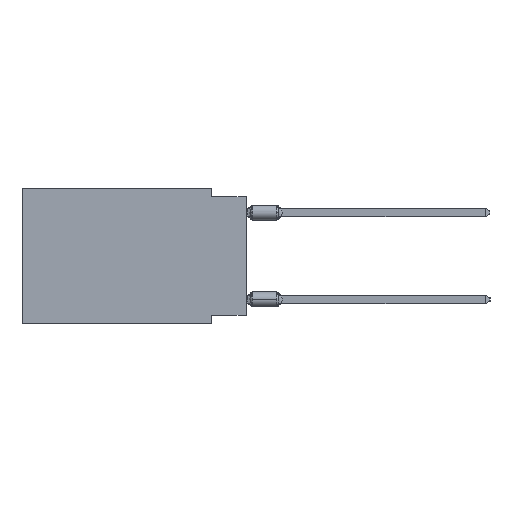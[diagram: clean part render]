
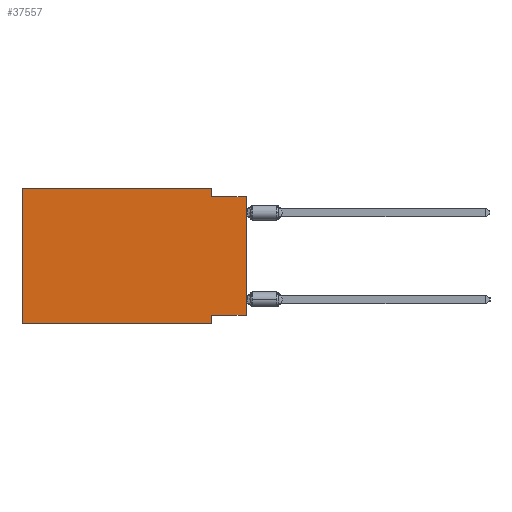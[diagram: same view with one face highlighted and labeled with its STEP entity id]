
A CAD part, left-side view. The second image highlights one B-rep face of the part: STEP entity #37557.
In plain terms, the highlighted planar face has unit normal (-1, 0, 0).
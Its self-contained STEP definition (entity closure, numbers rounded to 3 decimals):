
#1006 = VECTOR ( 'NONE', #11086, 1000. ) ;
#1692 = VECTOR ( 'NONE', #4965, 1000. ) ;
#1946 = PLANE ( 'NONE',  #30119 ) ;
#2645 = LINE ( 'NONE', #5754, #31853 ) ;
#2803 = CARTESIAN_POINT ( 'NONE',  ( 0., 16.383, 0. ) ) ;
#3024 = EDGE_CURVE ( 'NONE', #30024, #15613, #28320, .T. ) ;
#3860 = CARTESIAN_POINT ( 'NONE',  ( 0., 2.54, -9.271 ) ) ;
#4037 = DIRECTION ( 'NONE',  ( 0., 1., 0. ) ) ;
#4965 = DIRECTION ( 'NONE',  ( 0., 0., 1. ) ) ;
#5754 = CARTESIAN_POINT ( 'NONE',  ( 0., 0., -0.635 ) ) ;
#6241 = ORIENTED_EDGE ( 'NONE', *, *, #9407, .F. ) ;
#6508 = VECTOR ( 'NONE', #21291, 1000. ) ;
#6972 = ORIENTED_EDGE ( 'NONE', *, *, #30309, .F. ) ;
#7130 = ORIENTED_EDGE ( 'NONE', *, *, #29194, .T. ) ;
#7283 = VERTEX_POINT ( 'NONE', #7857 ) ;
#7857 = CARTESIAN_POINT ( 'NONE',  ( 0., 16.383, 0. ) ) ;
#8358 = VERTEX_POINT ( 'NONE', #12659 ) ;
#8396 = VECTOR ( 'NONE', #17007, 1000. ) ;
#8536 = DIRECTION ( 'NONE',  ( 1., 0., 0. ) ) ;
#8633 = EDGE_LOOP ( 'NONE', ( #27530, #24443, #30671, #10211, #6972, #7130, #30301, #6241 ) ) ;
#9407 = EDGE_CURVE ( 'NONE', #30024, #36001, #18699, .T. ) ;
#10211 = ORIENTED_EDGE ( 'NONE', *, *, #33633, .F. ) ;
#11086 = DIRECTION ( 'NONE',  ( 0., 0., 1. ) ) ;
#11648 = CARTESIAN_POINT ( 'NONE',  ( 0., 2.54, -0.635 ) ) ;
#12659 = CARTESIAN_POINT ( 'NONE',  ( 0., 16.383, -9.906 ) ) ;
#14315 = FACE_OUTER_BOUND ( 'NONE', #8633, .T. ) ;
#14510 = CARTESIAN_POINT ( 'NONE',  ( 0., 16.383, 0. ) ) ;
#14517 = VECTOR ( 'NONE', #34307, 1000. ) ;
#14641 = DIRECTION ( 'NONE',  ( 0., -1., 0. ) ) ;
#15522 = VERTEX_POINT ( 'NONE', #22913 ) ;
#15613 = VERTEX_POINT ( 'NONE', #26211 ) ;
#17007 = DIRECTION ( 'NONE',  ( 0., 0., -1. ) ) ;
#17102 = EDGE_CURVE ( 'NONE', #15522, #23818, #37337, .T. ) ;
#17480 = CARTESIAN_POINT ( 'NONE',  ( 0., 0., -9.271 ) ) ;
#18672 = CARTESIAN_POINT ( 'NONE',  ( 0., 2.54, -9.906 ) ) ;
#18699 = LINE ( 'NONE', #23718, #21127 ) ;
#19185 = CARTESIAN_POINT ( 'NONE',  ( 0., 2.54, 0. ) ) ;
#19701 = LINE ( 'NONE', #32058, #8396 ) ;
#21127 = VECTOR ( 'NONE', #4037, 1000. ) ;
#21291 = DIRECTION ( 'NONE',  ( 0., -1., 0. ) ) ;
#22701 = CARTESIAN_POINT ( 'NONE',  ( 0., 0., 0. ) ) ;
#22913 = CARTESIAN_POINT ( 'NONE',  ( 0., 2.54, 0. ) ) ;
#23718 = CARTESIAN_POINT ( 'NONE',  ( 0., 0., -9.271 ) ) ;
#23818 = VERTEX_POINT ( 'NONE', #11648 ) ;
#24443 = ORIENTED_EDGE ( 'NONE', *, *, #35143, .F. ) ;
#24567 = LINE ( 'NONE', #32692, #6508 ) ;
#25624 = VECTOR ( 'NONE', #27879, 1000. ) ;
#26211 = CARTESIAN_POINT ( 'NONE',  ( 0., 0., -0.635 ) ) ;
#27530 = ORIENTED_EDGE ( 'NONE', *, *, #3024, .T. ) ;
#27879 = DIRECTION ( 'NONE',  ( 0., 0., -1. ) ) ;
#28320 = LINE ( 'NONE', #22701, #1692 ) ;
#28985 = DIRECTION ( 'NONE',  ( 0., 0., -1. ) ) ;
#29194 = EDGE_CURVE ( 'NONE', #8358, #29672, #24567, .T. ) ;
#29672 = VERTEX_POINT ( 'NONE', #18672 ) ;
#30024 = VERTEX_POINT ( 'NONE', #17480 ) ;
#30119 = AXIS2_PLACEMENT_3D ( 'NONE', #14510, #8536, #28985 ) ;
#30301 = ORIENTED_EDGE ( 'NONE', *, *, #31556, .F. ) ;
#30309 = EDGE_CURVE ( 'NONE', #8358, #7283, #34631, .T. ) ;
#30671 = ORIENTED_EDGE ( 'NONE', *, *, #17102, .F. ) ;
#31556 = EDGE_CURVE ( 'NONE', #36001, #29672, #19701, .T. ) ;
#31853 = VECTOR ( 'NONE', #14641, 1000. ) ;
#32058 = CARTESIAN_POINT ( 'NONE',  ( 0., 2.54, -9.906 ) ) ;
#32692 = CARTESIAN_POINT ( 'NONE',  ( 0., 16.383, -9.906 ) ) ;
#33633 = EDGE_CURVE ( 'NONE', #7283, #15522, #35064, .T. ) ;
#34307 = DIRECTION ( 'NONE',  ( 0., -1., 0. ) ) ;
#34631 = LINE ( 'NONE', #37539, #1006 ) ;
#35064 = LINE ( 'NONE', #2803, #14517 ) ;
#35143 = EDGE_CURVE ( 'NONE', #23818, #15613, #2645, .T. ) ;
#36001 = VERTEX_POINT ( 'NONE', #3860 ) ;
#37337 = LINE ( 'NONE', #19185, #25624 ) ;
#37539 = CARTESIAN_POINT ( 'NONE',  ( 0., 16.383, 0. ) ) ;
#37557 = ADVANCED_FACE ( 'NONE', ( #14315 ), #1946, .F. ) ;
